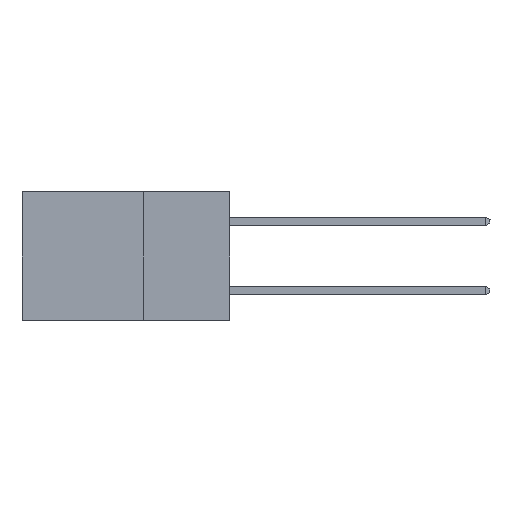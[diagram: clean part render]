
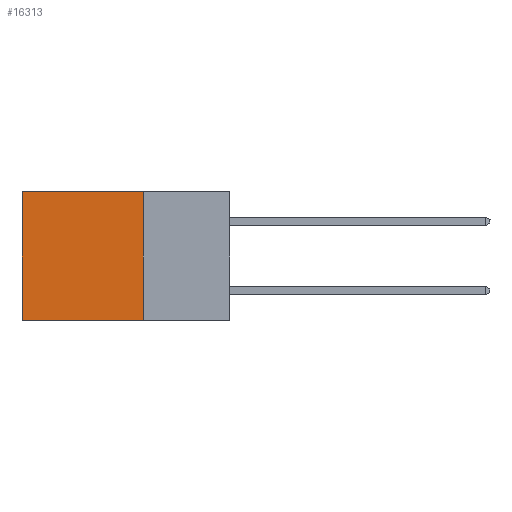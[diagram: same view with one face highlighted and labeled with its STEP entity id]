
A CAD part, left-side view. The second image highlights one B-rep face of the part: STEP entity #16313.
In plain terms, the highlighted planar face has unit normal (-1, 0, 0).
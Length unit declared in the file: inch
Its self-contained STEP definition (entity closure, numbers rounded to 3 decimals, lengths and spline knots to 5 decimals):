
#110 = EDGE_CURVE ( 'NONE', #6112, #9710, #5168, .T. ) ;
#2509 = VECTOR ( 'NONE', #5407, 39.37008 ) ;
#2549 = EDGE_LOOP ( 'NONE', ( #9813, #7619, #3448, #15746 ) ) ;
#3019 = CARTESIAN_POINT ( 'NONE',  ( 0.2615, 0.25, -0.37 ) ) ;
#3448 = ORIENTED_EDGE ( 'NONE', *, *, #8776, .F. ) ;
#3945 = DIRECTION ( 'NONE',  ( 1., 0., 0. ) ) ;
#5018 = CARTESIAN_POINT ( 'NONE',  ( 0.2615, 0.25, 0. ) ) ;
#5053 = CARTESIAN_POINT ( 'NONE',  ( 0.2615, 0.25, 0. ) ) ;
#5137 = VECTOR ( 'NONE', #21110, 39.37008 ) ;
#5168 = LINE ( 'NONE', #17529, #5137 ) ;
#5407 = DIRECTION ( 'NONE',  ( 0., 0., -1. ) ) ;
#5697 = PLANE ( 'NONE',  #12749 ) ;
#6112 = VERTEX_POINT ( 'NONE', #18954 ) ;
#6648 = LINE ( 'NONE', #5018, #17774 ) ;
#7619 = ORIENTED_EDGE ( 'NONE', *, *, #110, .F. ) ;
#7925 = EDGE_CURVE ( 'NONE', #22697, #9710, #16480, .T. ) ;
#8776 = EDGE_CURVE ( 'NONE', #21243, #6112, #12110, .T. ) ;
#9710 = VERTEX_POINT ( 'NONE', #18301 ) ;
#9813 = ORIENTED_EDGE ( 'NONE', *, *, #7925, .T. ) ;
#9957 = EDGE_CURVE ( 'NONE', #21243, #22697, #6648, .T. ) ;
#10939 = DIRECTION ( 'NONE',  ( 0., 0., -1. ) ) ;
#12110 = LINE ( 'NONE', #3019, #14094 ) ;
#12688 = FACE_OUTER_BOUND ( 'NONE', #2549, .T. ) ;
#12738 = CARTESIAN_POINT ( 'NONE',  ( 0.2615, 0.6, 0. ) ) ;
#12749 = AXIS2_PLACEMENT_3D ( 'NONE', #16303, #3945, #10939 ) ;
#14094 = VECTOR ( 'NONE', #19201, 39.37008 ) ;
#14109 = DIRECTION ( 'NONE',  ( 0., 1., 0. ) ) ;
#15746 = ORIENTED_EDGE ( 'NONE', *, *, #9957, .T. ) ;
#16303 = CARTESIAN_POINT ( 'NONE',  ( 0.2615, 0.25, -0.37 ) ) ;
#16313 = ADVANCED_FACE ( 'NONE', ( #12688 ), #5697, .F. ) ;
#16480 = LINE ( 'NONE', #21800, #2509 ) ;
#17529 = CARTESIAN_POINT ( 'NONE',  ( 0.2615, 0.25, -0.37 ) ) ;
#17774 = VECTOR ( 'NONE', #14109, 39.37008 ) ;
#18301 = CARTESIAN_POINT ( 'NONE',  ( 0.2615, 0.6, -0.37 ) ) ;
#18954 = CARTESIAN_POINT ( 'NONE',  ( 0.2615, 0.25, -0.37 ) ) ;
#19201 = DIRECTION ( 'NONE',  ( 0., 0., -1. ) ) ;
#21110 = DIRECTION ( 'NONE',  ( 0., 1., 0. ) ) ;
#21243 = VERTEX_POINT ( 'NONE', #5053 ) ;
#21800 = CARTESIAN_POINT ( 'NONE',  ( 0.2615, 0.6, -0.37 ) ) ;
#22697 = VERTEX_POINT ( 'NONE', #12738 ) ;
